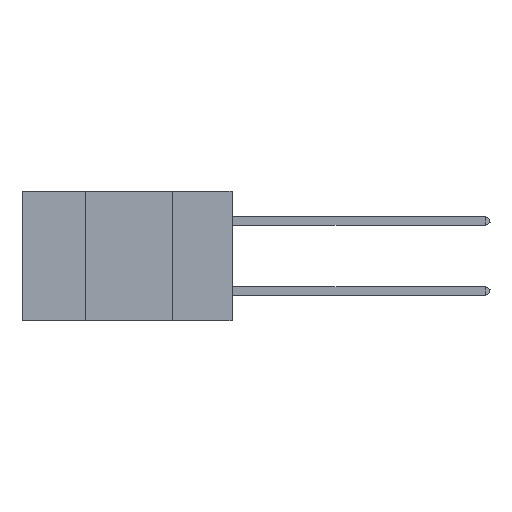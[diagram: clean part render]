
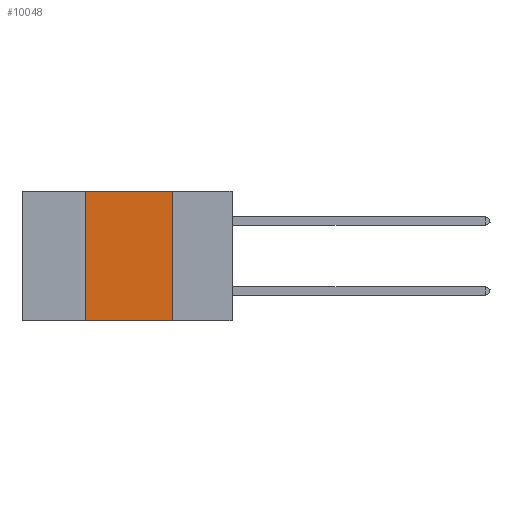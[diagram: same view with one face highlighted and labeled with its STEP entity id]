
A CAD part, left-side view. The second image highlights one B-rep face of the part: STEP entity #10048.
In plain terms, the highlighted planar face has unit normal (-1, 0, 0).
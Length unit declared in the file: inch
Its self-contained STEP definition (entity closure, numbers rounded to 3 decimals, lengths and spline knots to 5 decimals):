
#242 = CARTESIAN_POINT ( 'NONE',  ( 0., 0.42, 0. ) ) ;
#1019 = FACE_OUTER_BOUND ( 'NONE', #15209, .T. ) ;
#1736 = CARTESIAN_POINT ( 'NONE',  ( 0., 0.17, -0.37 ) ) ;
#2020 = CARTESIAN_POINT ( 'NONE',  ( 0., 0.6, 0. ) ) ;
#2928 = PLANE ( 'NONE',  #11070 ) ;
#2975 = CARTESIAN_POINT ( 'NONE',  ( 0., 0.6, -0.37 ) ) ;
#3034 = DIRECTION ( 'NONE',  ( 0., -1., 0. ) ) ;
#3931 = LINE ( 'NONE', #4979, #7054 ) ;
#4159 = ORIENTED_EDGE ( 'NONE', *, *, #15021, .F. ) ;
#4279 = CARTESIAN_POINT ( 'NONE',  ( 0., 0.6, 0. ) ) ;
#4605 = CARTESIAN_POINT ( 'NONE',  ( 0., 0.42, -0.37 ) ) ;
#4979 = CARTESIAN_POINT ( 'NONE',  ( 0., 0.17, 0. ) ) ;
#6329 = DIRECTION ( 'NONE',  ( 0., 0., -1. ) ) ;
#6440 = VECTOR ( 'NONE', #11270, 39.37008 ) ;
#6802 = VECTOR ( 'NONE', #3034, 39.37008 ) ;
#6950 = DIRECTION ( 'NONE',  ( 0., 0., -1. ) ) ;
#6999 = VERTEX_POINT ( 'NONE', #4605 ) ;
#7054 = VECTOR ( 'NONE', #6329, 39.37008 ) ;
#7180 = CARTESIAN_POINT ( 'NONE',  ( 0., 0.17, 0. ) ) ;
#7214 = LINE ( 'NONE', #2975, #6802 ) ;
#7606 = VERTEX_POINT ( 'NONE', #7180 ) ;
#8171 = EDGE_CURVE ( 'NONE', #6999, #9523, #7214, .T. ) ;
#9108 = VERTEX_POINT ( 'NONE', #13868 ) ;
#9523 = VERTEX_POINT ( 'NONE', #1736 ) ;
#10048 = ADVANCED_FACE ( 'NONE', ( #1019 ), #2928, .F. ) ;
#10777 = EDGE_CURVE ( 'NONE', #6999, #9108, #13236, .T. ) ;
#11070 = AXIS2_PLACEMENT_3D ( 'NONE', #4279, #14761, #6950 ) ;
#11270 = DIRECTION ( 'NONE',  ( 0., -1., 0. ) ) ;
#13236 = LINE ( 'NONE', #242, #16709 ) ;
#13868 = CARTESIAN_POINT ( 'NONE',  ( 0., 0.42, 0. ) ) ;
#14200 = ORIENTED_EDGE ( 'NONE', *, *, #15169, .F. ) ;
#14614 = ORIENTED_EDGE ( 'NONE', *, *, #10777, .F. ) ;
#14761 = DIRECTION ( 'NONE',  ( 1., 0., 0. ) ) ;
#15021 = EDGE_CURVE ( 'NONE', #9108, #7606, #16032, .T. ) ;
#15039 = ORIENTED_EDGE ( 'NONE', *, *, #8171, .T. ) ;
#15169 = EDGE_CURVE ( 'NONE', #7606, #9523, #3931, .T. ) ;
#15209 = EDGE_LOOP ( 'NONE', ( #14200, #4159, #14614, #15039 ) ) ;
#16032 = LINE ( 'NONE', #2020, #6440 ) ;
#16168 = DIRECTION ( 'NONE',  ( 0., 0., 1. ) ) ;
#16709 = VECTOR ( 'NONE', #16168, 39.37008 ) ;
